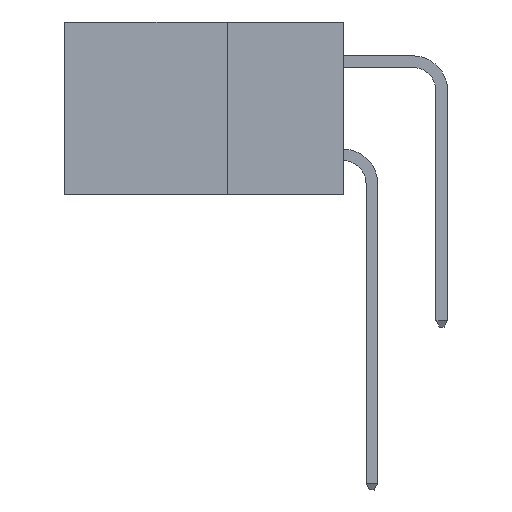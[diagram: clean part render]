
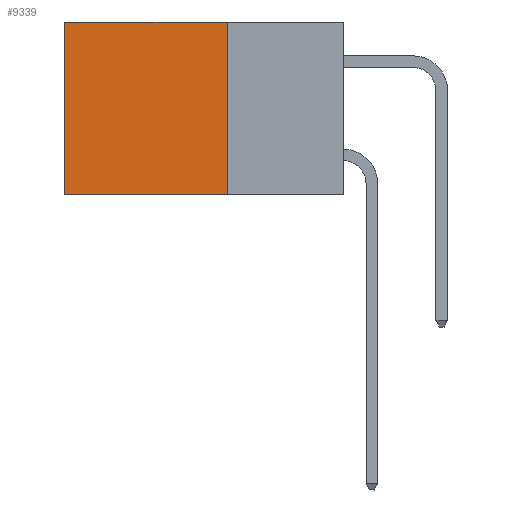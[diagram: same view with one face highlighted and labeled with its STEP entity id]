
A CAD part, left-side view. The second image highlights one B-rep face of the part: STEP entity #9339.
In plain terms, the highlighted planar face has unit normal (-1, 0, 0).
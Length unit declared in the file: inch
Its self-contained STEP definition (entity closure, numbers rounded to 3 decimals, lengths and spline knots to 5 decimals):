
#760 = FACE_OUTER_BOUND ( 'NONE', #9495, .T. ) ;
#2036 = DIRECTION ( 'NONE',  ( 0., 1., 0. ) ) ;
#2107 = CARTESIAN_POINT ( 'NONE',  ( 0.298, 0.25, -0.37 ) ) ;
#2269 = CARTESIAN_POINT ( 'NONE',  ( 0.298, 0.25, 0. ) ) ;
#2484 = EDGE_CURVE ( 'NONE', #11648, #6199, #12790, .T. ) ;
#2861 = ORIENTED_EDGE ( 'NONE', *, *, #15128, .T. ) ;
#2964 = ORIENTED_EDGE ( 'NONE', *, *, #17698, .F. ) ;
#3243 = CARTESIAN_POINT ( 'NONE',  ( 0.298, 0.6, 0. ) ) ;
#4299 = VECTOR ( 'NONE', #11751, 39.37008 ) ;
#5582 = AXIS2_PLACEMENT_3D ( 'NONE', #16353, #9068, #6365 ) ;
#6199 = VERTEX_POINT ( 'NONE', #3243 ) ;
#6365 = DIRECTION ( 'NONE',  ( 0., 0., -1. ) ) ;
#6609 = DIRECTION ( 'NONE',  ( 0., 0., -1. ) ) ;
#7433 = CARTESIAN_POINT ( 'NONE',  ( 0.298, 0.25, 0. ) ) ;
#7564 = PLANE ( 'NONE',  #5582 ) ;
#7791 = VECTOR ( 'NONE', #2036, 39.37008 ) ;
#8261 = CARTESIAN_POINT ( 'NONE',  ( 0.298, 0.6, -0.37 ) ) ;
#8610 = VERTEX_POINT ( 'NONE', #9906 ) ;
#9000 = VERTEX_POINT ( 'NONE', #8261 ) ;
#9068 = DIRECTION ( 'NONE',  ( 1., 0., 0. ) ) ;
#9309 = VECTOR ( 'NONE', #6609, 39.37008 ) ;
#9339 = ADVANCED_FACE ( 'NONE', ( #760 ), #7564, .F. ) ;
#9495 = EDGE_LOOP ( 'NONE', ( #2861, #9679, #2964, #15585 ) ) ;
#9640 = CARTESIAN_POINT ( 'NONE',  ( 0.298, 0.6, 0. ) ) ;
#9679 = ORIENTED_EDGE ( 'NONE', *, *, #10023, .F. ) ;
#9906 = CARTESIAN_POINT ( 'NONE',  ( 0.298, 0.25, -0.37 ) ) ;
#10023 = EDGE_CURVE ( 'NONE', #8610, #9000, #15668, .T. ) ;
#11147 = LINE ( 'NONE', #9640, #9309 ) ;
#11571 = VECTOR ( 'NONE', #16914, 39.37008 ) ;
#11648 = VERTEX_POINT ( 'NONE', #2269 ) ;
#11751 = DIRECTION ( 'NONE',  ( 0., 0., -1. ) ) ;
#12790 = LINE ( 'NONE', #18052, #7791 ) ;
#15128 = EDGE_CURVE ( 'NONE', #6199, #9000, #11147, .T. ) ;
#15585 = ORIENTED_EDGE ( 'NONE', *, *, #2484, .T. ) ;
#15668 = LINE ( 'NONE', #2107, #11571 ) ;
#16116 = LINE ( 'NONE', #7433, #4299 ) ;
#16353 = CARTESIAN_POINT ( 'NONE',  ( 0.298, 0.25, 0. ) ) ;
#16914 = DIRECTION ( 'NONE',  ( 0., 1., 0. ) ) ;
#17698 = EDGE_CURVE ( 'NONE', #11648, #8610, #16116, .T. ) ;
#18052 = CARTESIAN_POINT ( 'NONE',  ( 0.298, 0.25, 0. ) ) ;
